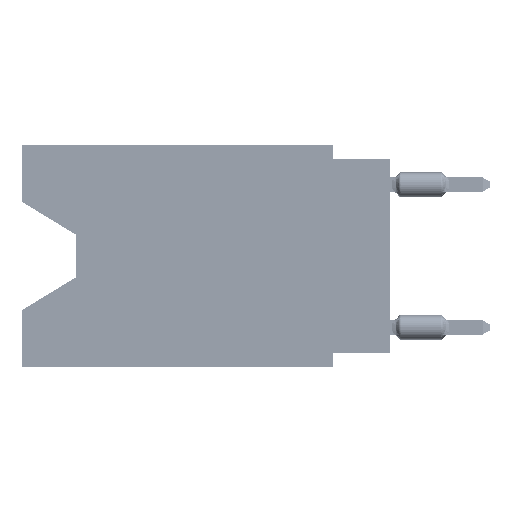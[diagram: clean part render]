
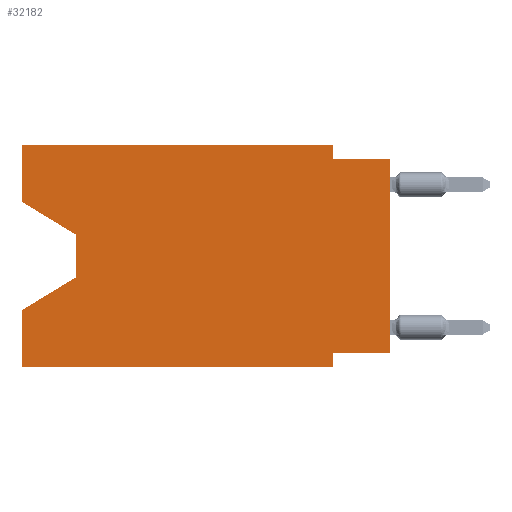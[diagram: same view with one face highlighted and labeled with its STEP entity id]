
A CAD part, left-side view. The second image highlights one B-rep face of the part: STEP entity #32182.
In plain terms, the highlighted planar face has unit normal (-1, 0, 0).
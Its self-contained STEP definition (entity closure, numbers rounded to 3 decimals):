
#62 = VERTEX_POINT ( 'NONE', #7696 ) ;
#213 = CARTESIAN_POINT ( 'NONE',  ( 0., 0., 0. ) ) ;
#380 = LINE ( 'NONE', #11517, #62149 ) ;
#460 = EDGE_CURVE ( 'NONE', #67744, #62, #2238, .T. ) ;
#823 = ORIENTED_EDGE ( 'NONE', *, *, #41904, .F. ) ;
#947 = EDGE_CURVE ( 'NONE', #45037, #62, #39427, .T. ) ;
#1338 = VERTEX_POINT ( 'NONE', #43597 ) ;
#1753 = DIRECTION ( 'NONE',  ( 0., 0., -1. ) ) ;
#1972 = VECTOR ( 'NONE', #5912, 1000. ) ;
#2238 = LINE ( 'NONE', #36474, #2817 ) ;
#2817 = VECTOR ( 'NONE', #59964, 1000. ) ;
#4065 = VECTOR ( 'NONE', #72724, 1000. ) ;
#4586 = LINE ( 'NONE', #10340, #59949 ) ;
#5912 = DIRECTION ( 'NONE',  ( 0., 0.855, -0.519 ) ) ;
#6115 = EDGE_CURVE ( 'NONE', #74864, #19253, #41307, .T. ) ;
#6486 = VECTOR ( 'NONE', #62151, 1000. ) ;
#6706 = EDGE_CURVE ( 'NONE', #66602, #33450, #24069, .T. ) ;
#7342 = DIRECTION ( 'NONE',  ( 0., 0., 1. ) ) ;
#7696 = CARTESIAN_POINT ( 'NONE',  ( 0., 2.54, -9.906 ) ) ;
#7807 = CARTESIAN_POINT ( 'NONE',  ( 0., 0., -0.635 ) ) ;
#8463 = CARTESIAN_POINT ( 'NONE',  ( 0., 16.383, 0. ) ) ;
#8798 = CARTESIAN_POINT ( 'NONE',  ( 0., 16.383, 0. ) ) ;
#9796 = EDGE_CURVE ( 'NONE', #52524, #74864, #65998, .T. ) ;
#10340 = CARTESIAN_POINT ( 'NONE',  ( 0., 0., -9.271 ) ) ;
#11341 = PLANE ( 'NONE',  #69437 ) ;
#11517 = CARTESIAN_POINT ( 'NONE',  ( 0., 16.383, -2.546 ) ) ;
#11726 = DIRECTION ( 'NONE',  ( 0., 0., -1. ) ) ;
#14888 = CARTESIAN_POINT ( 'NONE',  ( 0., 16.383, -2.546 ) ) ;
#14940 = CARTESIAN_POINT ( 'NONE',  ( 0., 0., -9.271 ) ) ;
#16449 = VECTOR ( 'NONE', #43835, 1000. ) ;
#17718 = EDGE_CURVE ( 'NONE', #45037, #19253, #54276, .T. ) ;
#19253 = VERTEX_POINT ( 'NONE', #30411 ) ;
#20747 = LINE ( 'NONE', #8798, #16449 ) ;
#21814 = VECTOR ( 'NONE', #1753, 1000. ) ;
#21997 = CARTESIAN_POINT ( 'NONE',  ( 0., 2.54, -0.635 ) ) ;
#24069 = LINE ( 'NONE', #213, #54867 ) ;
#24236 = DIRECTION ( 'NONE',  ( 0., -0.855, -0.519 ) ) ;
#27039 = EDGE_CURVE ( 'NONE', #1338, #69703, #56577, .T. ) ;
#27675 = CARTESIAN_POINT ( 'NONE',  ( 0., 16.383, -9.906 ) ) ;
#29915 = EDGE_LOOP ( 'NONE', ( #30459, #47766, #58556, #64795, #45330, #53051, #823, #69801, #48626, #38581, #75089, #70955 ) ) ;
#30248 = CARTESIAN_POINT ( 'NONE',  ( 0., 13.97, -4.013 ) ) ;
#30411 = CARTESIAN_POINT ( 'NONE',  ( 0., 16.383, -7.36 ) ) ;
#30459 = ORIENTED_EDGE ( 'NONE', *, *, #66327, .T. ) ;
#32182 = ADVANCED_FACE ( 'NONE', ( #65583 ), #11341, .F. ) ;
#33450 = VERTEX_POINT ( 'NONE', #47540 ) ;
#33805 = DIRECTION ( 'NONE',  ( 0., 1., 0. ) ) ;
#36193 = CARTESIAN_POINT ( 'NONE',  ( 0., 16.383, 0. ) ) ;
#36474 = CARTESIAN_POINT ( 'NONE',  ( 0., 2.54, -9.906 ) ) ;
#37698 = LINE ( 'NONE', #8463, #40159 ) ;
#38580 = DIRECTION ( 'NONE',  ( 0., -1., 0. ) ) ;
#38581 = ORIENTED_EDGE ( 'NONE', *, *, #27039, .F. ) ;
#39427 = LINE ( 'NONE', #62895, #6486 ) ;
#40159 = VECTOR ( 'NONE', #68459, 1000. ) ;
#40549 = CARTESIAN_POINT ( 'NONE',  ( 0., 13.97, -5.893 ) ) ;
#41307 = LINE ( 'NONE', #40549, #1972 ) ;
#41367 = DIRECTION ( 'NONE',  ( 1., 0., 0. ) ) ;
#41904 = EDGE_CURVE ( 'NONE', #66602, #67744, #4586, .T. ) ;
#43597 = CARTESIAN_POINT ( 'NONE',  ( 0., 2.54, 0. ) ) ;
#43835 = DIRECTION ( 'NONE',  ( 0., 0., 1. ) ) ;
#44279 = CARTESIAN_POINT ( 'NONE',  ( 0., 2.54, 0. ) ) ;
#45037 = VERTEX_POINT ( 'NONE', #27675 ) ;
#45330 = ORIENTED_EDGE ( 'NONE', *, *, #947, .T. ) ;
#47540 = CARTESIAN_POINT ( 'NONE',  ( 0., 0., -0.635 ) ) ;
#47766 = ORIENTED_EDGE ( 'NONE', *, *, #9796, .T. ) ;
#48626 = ORIENTED_EDGE ( 'NONE', *, *, #58644, .F. ) ;
#49216 = CARTESIAN_POINT ( 'NONE',  ( 0., 2.54, -9.271 ) ) ;
#50034 = VECTOR ( 'NONE', #7342, 1000. ) ;
#50913 = EDGE_CURVE ( 'NONE', #70577, #61154, #20747, .T. ) ;
#52524 = VERTEX_POINT ( 'NONE', #71923 ) ;
#53051 = ORIENTED_EDGE ( 'NONE', *, *, #460, .F. ) ;
#54276 = LINE ( 'NONE', #36193, #50034 ) ;
#54526 = EDGE_CURVE ( 'NONE', #61154, #1338, #37698, .T. ) ;
#54588 = CARTESIAN_POINT ( 'NONE',  ( 0., 13.97, -5.893 ) ) ;
#54867 = VECTOR ( 'NONE', #76015, 1000. ) ;
#56577 = LINE ( 'NONE', #44279, #4065 ) ;
#57688 = VECTOR ( 'NONE', #38580, 1000. ) ;
#58556 = ORIENTED_EDGE ( 'NONE', *, *, #6115, .T. ) ;
#58644 = EDGE_CURVE ( 'NONE', #69703, #33450, #60526, .T. ) ;
#59949 = VECTOR ( 'NONE', #33805, 1000. ) ;
#59964 = DIRECTION ( 'NONE',  ( 0., 0., -1. ) ) ;
#60276 = CARTESIAN_POINT ( 'NONE',  ( 0., 16.383, 0. ) ) ;
#60526 = LINE ( 'NONE', #7807, #57688 ) ;
#61154 = VERTEX_POINT ( 'NONE', #60276 ) ;
#62149 = VECTOR ( 'NONE', #24236, 1000. ) ;
#62151 = DIRECTION ( 'NONE',  ( 0., -1., 0. ) ) ;
#62895 = CARTESIAN_POINT ( 'NONE',  ( 0., 16.383, -9.906 ) ) ;
#64795 = ORIENTED_EDGE ( 'NONE', *, *, #17718, .F. ) ;
#65583 = FACE_OUTER_BOUND ( 'NONE', #29915, .T. ) ;
#65998 = LINE ( 'NONE', #30248, #21814 ) ;
#66327 = EDGE_CURVE ( 'NONE', #70577, #52524, #380, .T. ) ;
#66602 = VERTEX_POINT ( 'NONE', #14940 ) ;
#67744 = VERTEX_POINT ( 'NONE', #49216 ) ;
#68459 = DIRECTION ( 'NONE',  ( 0., -1., 0. ) ) ;
#69437 = AXIS2_PLACEMENT_3D ( 'NONE', #76002, #41367, #11726 ) ;
#69703 = VERTEX_POINT ( 'NONE', #21997 ) ;
#69801 = ORIENTED_EDGE ( 'NONE', *, *, #6706, .T. ) ;
#70577 = VERTEX_POINT ( 'NONE', #14888 ) ;
#70955 = ORIENTED_EDGE ( 'NONE', *, *, #50913, .F. ) ;
#71923 = CARTESIAN_POINT ( 'NONE',  ( 0., 13.97, -4.013 ) ) ;
#72724 = DIRECTION ( 'NONE',  ( 0., 0., -1. ) ) ;
#74864 = VERTEX_POINT ( 'NONE', #54588 ) ;
#75089 = ORIENTED_EDGE ( 'NONE', *, *, #54526, .F. ) ;
#76002 = CARTESIAN_POINT ( 'NONE',  ( 0., 16.383, 0. ) ) ;
#76015 = DIRECTION ( 'NONE',  ( 0., 0., 1. ) ) ;
